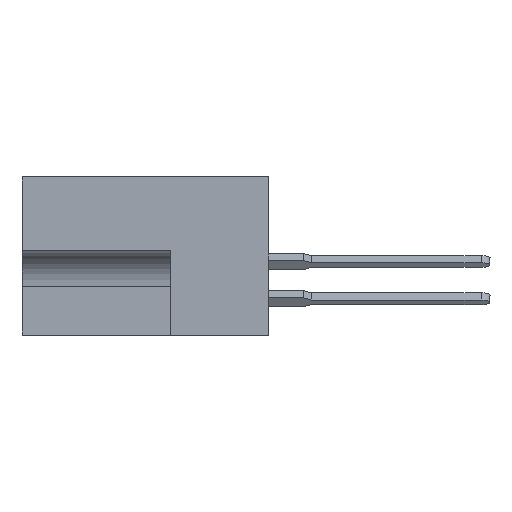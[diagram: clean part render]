
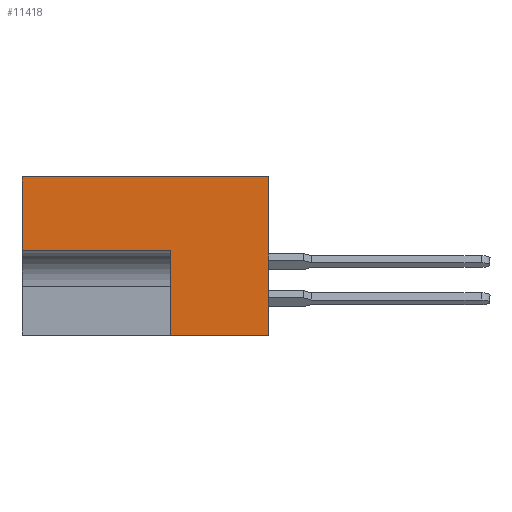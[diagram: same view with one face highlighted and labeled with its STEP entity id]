
A CAD part, left-side view. The second image highlights one B-rep face of the part: STEP entity #11418.
In plain terms, the highlighted planar face has unit normal (-1, 0, 0).
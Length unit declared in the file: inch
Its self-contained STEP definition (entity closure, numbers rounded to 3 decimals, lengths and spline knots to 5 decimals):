
#28 = CARTESIAN_POINT ( 'NONE',  ( 0., 0., 0. ) ) ;
#38 = PLANE ( 'NONE',  #17665 ) ;
#114 = VERTEX_POINT ( 'NONE', #9694 ) ;
#298 = DIRECTION ( 'NONE',  ( 0., 0., 1. ) ) ;
#454 = EDGE_CURVE ( 'NONE', #9184, #6635, #19275, .T. ) ;
#914 = VERTEX_POINT ( 'NONE', #18194 ) ;
#942 = VECTOR ( 'NONE', #17564, 39.37008 ) ;
#1235 = VECTOR ( 'NONE', #12761, 39.37008 ) ;
#2383 = ORIENTED_EDGE ( 'NONE', *, *, #16366, .F. ) ;
#2522 = EDGE_CURVE ( 'NONE', #114, #6635, #17986, .T. ) ;
#2859 = DIRECTION ( 'NONE',  ( 0., 0., 1. ) ) ;
#3076 = CARTESIAN_POINT ( 'NONE',  ( 0., 0.453, 0. ) ) ;
#3138 = ORIENTED_EDGE ( 'NONE', *, *, #4893, .F. ) ;
#4218 = CARTESIAN_POINT ( 'NONE',  ( 0., 0.828, 0. ) ) ;
#4630 = VECTOR ( 'NONE', #2859, 39.37008 ) ;
#4844 = LINE ( 'NONE', #5918, #4630 ) ;
#4863 = CARTESIAN_POINT ( 'NONE',  ( 0., 0.328, -0.248 ) ) ;
#4893 = EDGE_CURVE ( 'NONE', #914, #16706, #4844, .T. ) ;
#5736 = CARTESIAN_POINT ( 'NONE',  ( 0., 0.328, -0.248 ) ) ;
#5918 = CARTESIAN_POINT ( 'NONE',  ( 0., 0.328, -0.531 ) ) ;
#6635 = VERTEX_POINT ( 'NONE', #17092 ) ;
#7052 = FACE_OUTER_BOUND ( 'NONE', #12962, .T. ) ;
#7398 = EDGE_CURVE ( 'NONE', #16706, #13591, #9069, .T. ) ;
#7535 = DIRECTION ( 'NONE',  ( 1., 0., 0. ) ) ;
#8107 = VECTOR ( 'NONE', #18738, 39.37008 ) ;
#9069 = LINE ( 'NONE', #4863, #1235 ) ;
#9184 = VERTEX_POINT ( 'NONE', #4218 ) ;
#9694 = CARTESIAN_POINT ( 'NONE',  ( 0., 0., -0.531 ) ) ;
#9923 = EDGE_CURVE ( 'NONE', #914, #114, #11196, .T. ) ;
#10549 = CARTESIAN_POINT ( 'NONE',  ( 0., 0.828, -0.248 ) ) ;
#11196 = LINE ( 'NONE', #13869, #14985 ) ;
#11370 = CARTESIAN_POINT ( 'NONE',  ( 0., 0.828, 0. ) ) ;
#11418 = ADVANCED_FACE ( 'NONE', ( #7052 ), #38, .F. ) ;
#11980 = DIRECTION ( 'NONE',  ( 0., 0., -1. ) ) ;
#12519 = VECTOR ( 'NONE', #298, 39.37008 ) ;
#12761 = DIRECTION ( 'NONE',  ( 0., 1., 0. ) ) ;
#12962 = EDGE_LOOP ( 'NONE', ( #2383, #19224, #3138, #16668, #14392, #16683 ) ) ;
#13045 = CARTESIAN_POINT ( 'NONE',  ( 0., 0.453, 0. ) ) ;
#13591 = VERTEX_POINT ( 'NONE', #10549 ) ;
#13869 = CARTESIAN_POINT ( 'NONE',  ( 0., 0.453, -0.531 ) ) ;
#14392 = ORIENTED_EDGE ( 'NONE', *, *, #2522, .T. ) ;
#14985 = VECTOR ( 'NONE', #18644, 39.37008 ) ;
#16366 = EDGE_CURVE ( 'NONE', #13591, #9184, #17890, .T. ) ;
#16668 = ORIENTED_EDGE ( 'NONE', *, *, #9923, .T. ) ;
#16683 = ORIENTED_EDGE ( 'NONE', *, *, #454, .F. ) ;
#16706 = VERTEX_POINT ( 'NONE', #5736 ) ;
#17092 = CARTESIAN_POINT ( 'NONE',  ( 0., 0., 0. ) ) ;
#17564 = DIRECTION ( 'NONE',  ( 0., -1., 0. ) ) ;
#17665 = AXIS2_PLACEMENT_3D ( 'NONE', #3076, #7535, #11980 ) ;
#17890 = LINE ( 'NONE', #11370, #8107 ) ;
#17986 = LINE ( 'NONE', #28, #12519 ) ;
#18194 = CARTESIAN_POINT ( 'NONE',  ( 0., 0.328, -0.531 ) ) ;
#18644 = DIRECTION ( 'NONE',  ( 0., -1., 0. ) ) ;
#18738 = DIRECTION ( 'NONE',  ( 0., 0., 1. ) ) ;
#19224 = ORIENTED_EDGE ( 'NONE', *, *, #7398, .F. ) ;
#19275 = LINE ( 'NONE', #13045, #942 ) ;
